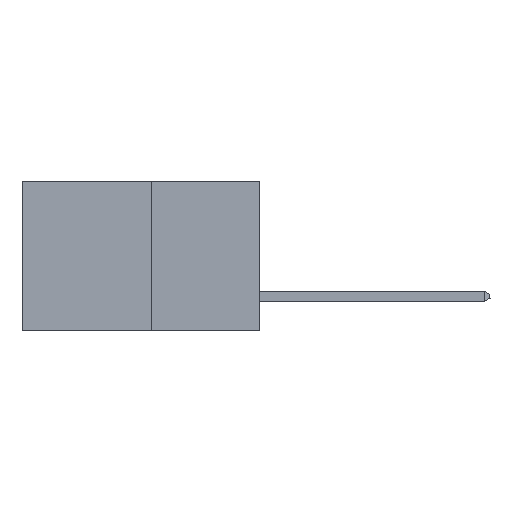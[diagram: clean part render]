
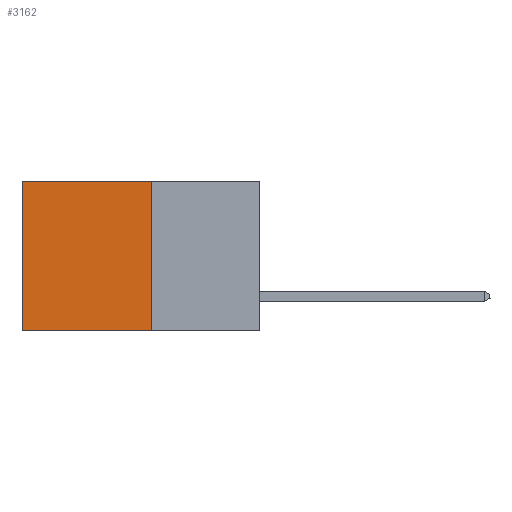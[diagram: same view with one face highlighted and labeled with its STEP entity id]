
A CAD part, left-side view. The second image highlights one B-rep face of the part: STEP entity #3162.
In plain terms, the highlighted planar face has unit normal (-1, 0, 0).
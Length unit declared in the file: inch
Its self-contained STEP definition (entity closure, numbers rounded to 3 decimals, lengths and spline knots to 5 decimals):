
#477 = ORIENTED_EDGE ( 'NONE', *, *, #4817, .T. ) ;
#926 = EDGE_CURVE ( 'NONE', #8541, #9585, #3452, .T. ) ;
#1555 = LINE ( 'NONE', #15347, #10900 ) ;
#1953 = AXIS2_PLACEMENT_3D ( 'NONE', #6013, #5493, #4906 ) ;
#2480 = VERTEX_POINT ( 'NONE', #11209 ) ;
#3162 = ADVANCED_FACE ( 'NONE', ( #11231 ), #6036, .F. ) ;
#3271 = DIRECTION ( 'NONE',  ( 0., 0., -1. ) ) ;
#3452 = LINE ( 'NONE', #6877, #15374 ) ;
#3697 = CARTESIAN_POINT ( 'NONE',  ( 0.277, 0.27, -0.37 ) ) ;
#4502 = CARTESIAN_POINT ( 'NONE',  ( 0.277, 0.27, -0.37 ) ) ;
#4817 = EDGE_CURVE ( 'NONE', #2480, #14922, #1555, .T. ) ;
#4906 = DIRECTION ( 'NONE',  ( 0., 0., -1. ) ) ;
#5153 = LINE ( 'NONE', #3697, #11127 ) ;
#5493 = DIRECTION ( 'NONE',  ( 1., 0., 0. ) ) ;
#5708 = LINE ( 'NONE', #12742, #14167 ) ;
#6013 = CARTESIAN_POINT ( 'NONE',  ( 0.277, 0.27, -0.37 ) ) ;
#6036 = PLANE ( 'NONE',  #1953 ) ;
#6877 = CARTESIAN_POINT ( 'NONE',  ( 0.277, 0.27, -0.37 ) ) ;
#6973 = EDGE_LOOP ( 'NONE', ( #9654, #12662, #10003, #477 ) ) ;
#8541 = VERTEX_POINT ( 'NONE', #4502 ) ;
#8629 = CARTESIAN_POINT ( 'NONE',  ( 0.277, 0.59, 0. ) ) ;
#8934 = CARTESIAN_POINT ( 'NONE',  ( 0.277, 0.59, -0.37 ) ) ;
#9427 = EDGE_CURVE ( 'NONE', #2480, #8541, #5153, .T. ) ;
#9585 = VERTEX_POINT ( 'NONE', #8934 ) ;
#9654 = ORIENTED_EDGE ( 'NONE', *, *, #12520, .T. ) ;
#10003 = ORIENTED_EDGE ( 'NONE', *, *, #9427, .F. ) ;
#10894 = DIRECTION ( 'NONE',  ( 0., 0., -1. ) ) ;
#10900 = VECTOR ( 'NONE', #15272, 39.37008 ) ;
#11127 = VECTOR ( 'NONE', #10894, 39.37008 ) ;
#11209 = CARTESIAN_POINT ( 'NONE',  ( 0.277, 0.27, 0. ) ) ;
#11231 = FACE_OUTER_BOUND ( 'NONE', #6973, .T. ) ;
#12520 = EDGE_CURVE ( 'NONE', #14922, #9585, #5708, .T. ) ;
#12662 = ORIENTED_EDGE ( 'NONE', *, *, #926, .F. ) ;
#12742 = CARTESIAN_POINT ( 'NONE',  ( 0.277, 0.59, -0.37 ) ) ;
#13305 = DIRECTION ( 'NONE',  ( 0., 1., 0. ) ) ;
#14167 = VECTOR ( 'NONE', #3271, 39.37008 ) ;
#14922 = VERTEX_POINT ( 'NONE', #8629 ) ;
#15272 = DIRECTION ( 'NONE',  ( 0., 1., 0. ) ) ;
#15347 = CARTESIAN_POINT ( 'NONE',  ( 0.277, 0.27, 0. ) ) ;
#15374 = VECTOR ( 'NONE', #13305, 39.37008 ) ;
